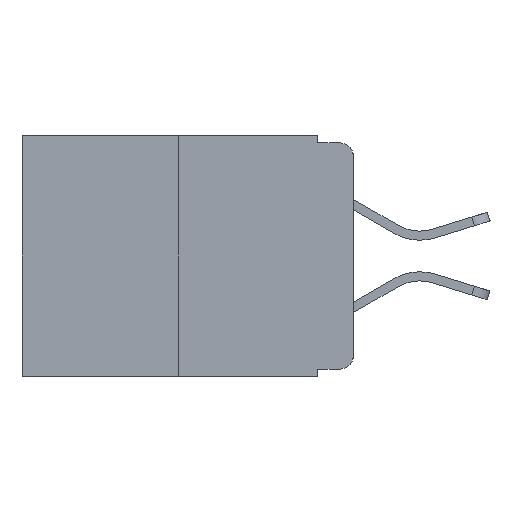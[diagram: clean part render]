
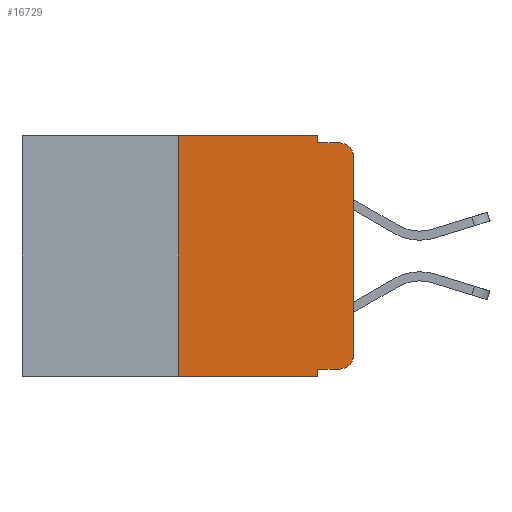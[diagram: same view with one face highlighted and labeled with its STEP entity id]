
A CAD part, left-side view. The second image highlights one B-rep face of the part: STEP entity #16729.
In plain terms, the highlighted planar face has unit normal (-1, 0, 0).
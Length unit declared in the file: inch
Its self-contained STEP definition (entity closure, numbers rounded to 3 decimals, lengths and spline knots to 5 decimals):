
#33 = EDGE_LOOP ( 'NONE', ( #16461, #3311, #4307, #6264, #2354, #10853, #13600, #18290, #1133, #5845 ) ) ;
#53 = VERTEX_POINT ( 'NONE', #7600 ) ;
#1133 = ORIENTED_EDGE ( 'NONE', *, *, #5441, .T. ) ;
#1193 = VECTOR ( 'NONE', #14844, 39.37008 ) ;
#1341 = VERTEX_POINT ( 'NONE', #18229 ) ;
#1594 = VERTEX_POINT ( 'NONE', #16532 ) ;
#1629 = LINE ( 'NONE', #16760, #9481 ) ;
#1716 = CARTESIAN_POINT ( 'NONE',  ( 0., 0.473, 0. ) ) ;
#2089 = VERTEX_POINT ( 'NONE', #19067 ) ;
#2120 = VERTEX_POINT ( 'NONE', #12433 ) ;
#2354 = ORIENTED_EDGE ( 'NONE', *, *, #10135, .F. ) ;
#2574 = EDGE_CURVE ( 'NONE', #1594, #2120, #19396, .T. ) ;
#2835 = VECTOR ( 'NONE', #4657, 39.37008 ) ;
#3251 = VECTOR ( 'NONE', #14759, 39.37008 ) ;
#3311 = ORIENTED_EDGE ( 'NONE', *, *, #12586, .T. ) ;
#3341 = DIRECTION ( 'NONE',  ( 0., 0., -1. ) ) ;
#3362 = EDGE_CURVE ( 'NONE', #10504, #53, #6790, .T. ) ;
#3668 = LINE ( 'NONE', #14537, #18995 ) ;
#4307 = ORIENTED_EDGE ( 'NONE', *, *, #11609, .F. ) ;
#4657 = DIRECTION ( 'NONE',  ( 0., -1., 0. ) ) ;
#4825 = VERTEX_POINT ( 'NONE', #13118 ) ;
#5150 = CARTESIAN_POINT ( 'NONE',  ( 0., 0.02, -0.03 ) ) ;
#5441 = EDGE_CURVE ( 'NONE', #7313, #10504, #3668, .T. ) ;
#5671 = AXIS2_PLACEMENT_3D ( 'NONE', #5150, #15618, #6733 ) ;
#5845 = ORIENTED_EDGE ( 'NONE', *, *, #3362, .T. ) ;
#5956 = VERTEX_POINT ( 'NONE', #8303 ) ;
#6264 = ORIENTED_EDGE ( 'NONE', *, *, #10624, .F. ) ;
#6494 = EDGE_CURVE ( 'NONE', #7313, #2120, #1629, .T. ) ;
#6626 = CARTESIAN_POINT ( 'NONE',  ( 0., 0.02, -0.313 ) ) ;
#6733 = DIRECTION ( 'NONE',  ( 0., 0., -1. ) ) ;
#6790 = CIRCLE ( 'NONE', #7979, 0.02 ) ;
#7313 = VERTEX_POINT ( 'NONE', #15660 ) ;
#7579 = EDGE_CURVE ( 'NONE', #1594, #17026, #12444, .T. ) ;
#7600 = CARTESIAN_POINT ( 'NONE',  ( 0., 0., -0.313 ) ) ;
#7979 = AXIS2_PLACEMENT_3D ( 'NONE', #6626, #16978, #8242 ) ;
#8006 = CARTESIAN_POINT ( 'NONE',  ( 0., 0., 0. ) ) ;
#8242 = DIRECTION ( 'NONE',  ( 0., 0., -1. ) ) ;
#8303 = CARTESIAN_POINT ( 'NONE',  ( 0., 0., -0.03 ) ) ;
#8423 = FACE_OUTER_BOUND ( 'NONE', #33, .T. ) ;
#8518 = VECTOR ( 'NONE', #10720, 39.37008 ) ;
#8561 = CARTESIAN_POINT ( 'NONE',  ( 0., 0.02, -0.333 ) ) ;
#8725 = DIRECTION ( 'NONE',  ( 0., -1., 0. ) ) ;
#9236 = CARTESIAN_POINT ( 'NONE',  ( 0., 0.25, 0. ) ) ;
#9481 = VECTOR ( 'NONE', #12493, 39.37008 ) ;
#9517 = DIRECTION ( 'NONE',  ( 0., 0., 1. ) ) ;
#10135 = EDGE_CURVE ( 'NONE', #17026, #1341, #12377, .T. ) ;
#10504 = VERTEX_POINT ( 'NONE', #8561 ) ;
#10624 = EDGE_CURVE ( 'NONE', #1341, #2089, #11435, .T. ) ;
#10720 = DIRECTION ( 'NONE',  ( 0., 0., 1. ) ) ;
#10724 = VECTOR ( 'NONE', #9517, 39.37008 ) ;
#10853 = ORIENTED_EDGE ( 'NONE', *, *, #7579, .F. ) ;
#10886 = DIRECTION ( 'NONE',  ( 0., -1., 0. ) ) ;
#11031 = PLANE ( 'NONE',  #17411 ) ;
#11435 = LINE ( 'NONE', #13325, #3251 ) ;
#11609 = EDGE_CURVE ( 'NONE', #2089, #4825, #13457, .T. ) ;
#12364 = CARTESIAN_POINT ( 'NONE',  ( 0., 0.473, -0.343 ) ) ;
#12377 = LINE ( 'NONE', #19398, #2835 ) ;
#12433 = CARTESIAN_POINT ( 'NONE',  ( 0., 0.051, -0.343 ) ) ;
#12444 = LINE ( 'NONE', #9236, #8518 ) ;
#12493 = DIRECTION ( 'NONE',  ( 0., 0., -1. ) ) ;
#12506 = DIRECTION ( 'NONE',  ( 1., 0., 0. ) ) ;
#12586 = EDGE_CURVE ( 'NONE', #5956, #4825, #17793, .T. ) ;
#13118 = CARTESIAN_POINT ( 'NONE',  ( 0., 0.02, -0.01 ) ) ;
#13325 = CARTESIAN_POINT ( 'NONE',  ( 0., 0.051, 0. ) ) ;
#13413 = CARTESIAN_POINT ( 'NONE',  ( 0., 0.051, -0.01 ) ) ;
#13457 = LINE ( 'NONE', #13413, #1193 ) ;
#13600 = ORIENTED_EDGE ( 'NONE', *, *, #2574, .T. ) ;
#14512 = EDGE_CURVE ( 'NONE', #53, #5956, #18370, .T. ) ;
#14537 = CARTESIAN_POINT ( 'NONE',  ( 0., 0.051, -0.333 ) ) ;
#14759 = DIRECTION ( 'NONE',  ( 0., 0., -1. ) ) ;
#14844 = DIRECTION ( 'NONE',  ( 0., -1., 0. ) ) ;
#15618 = DIRECTION ( 'NONE',  ( -1., 0., 0. ) ) ;
#15660 = CARTESIAN_POINT ( 'NONE',  ( 0., 0.051, -0.333 ) ) ;
#16461 = ORIENTED_EDGE ( 'NONE', *, *, #14512, .T. ) ;
#16532 = CARTESIAN_POINT ( 'NONE',  ( 0., 0.25, -0.343 ) ) ;
#16729 = ADVANCED_FACE ( 'NONE', ( #8423 ), #11031, .F. ) ;
#16760 = CARTESIAN_POINT ( 'NONE',  ( 0., 0.051, 0. ) ) ;
#16978 = DIRECTION ( 'NONE',  ( -1., 0., 0. ) ) ;
#17026 = VERTEX_POINT ( 'NONE', #17446 ) ;
#17411 = AXIS2_PLACEMENT_3D ( 'NONE', #1716, #12506, #3341 ) ;
#17446 = CARTESIAN_POINT ( 'NONE',  ( 0., 0.25, 0. ) ) ;
#17793 = CIRCLE ( 'NONE', #5671, 0.02 ) ;
#18229 = CARTESIAN_POINT ( 'NONE',  ( 0., 0.051, 0. ) ) ;
#18290 = ORIENTED_EDGE ( 'NONE', *, *, #6494, .F. ) ;
#18370 = LINE ( 'NONE', #8006, #10724 ) ;
#18934 = VECTOR ( 'NONE', #10886, 39.37008 ) ;
#18995 = VECTOR ( 'NONE', #8725, 39.37008 ) ;
#19067 = CARTESIAN_POINT ( 'NONE',  ( 0., 0.051, -0.01 ) ) ;
#19396 = LINE ( 'NONE', #12364, #18934 ) ;
#19398 = CARTESIAN_POINT ( 'NONE',  ( 0., 0.473, 0. ) ) ;
